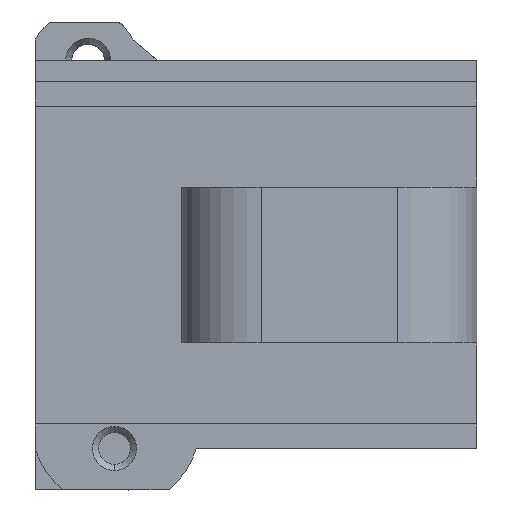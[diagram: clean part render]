
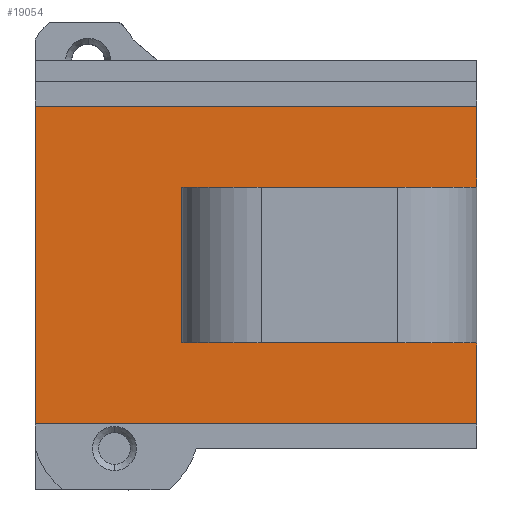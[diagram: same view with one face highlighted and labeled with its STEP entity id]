
A CAD part, left-side view. The second image highlights one B-rep face of the part: STEP entity #19054.
In plain terms, the highlighted planar face has unit normal (-1, 0, 0).
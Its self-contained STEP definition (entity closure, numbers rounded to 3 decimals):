
#2054 = DIRECTION ( 'NONE',  ( 0., 0., -1. ) ) ;
#2431 = VECTOR ( 'NONE', #35091, 1000. ) ;
#3809 = VERTEX_POINT ( 'NONE', #44843 ) ;
#7459 = LINE ( 'NONE', #10860, #109942 ) ;
#7646 = CARTESIAN_POINT ( 'NONE',  ( -40.849, 17.172, -13. ) ) ;
#8644 = DIRECTION ( 'NONE',  ( 0., 0., -1. ) ) ;
#9227 = EDGE_CURVE ( 'NONE', #20123, #62786, #75162, .T. ) ;
#9499 = VECTOR ( 'NONE', #72036, 1000. ) ;
#10860 = CARTESIAN_POINT ( 'NONE',  ( -40.849, 17.172, -13. ) ) ;
#11557 = ORIENTED_EDGE ( 'NONE', *, *, #70310, .F. ) ;
#17947 = VECTOR ( 'NONE', #8644, 1000. ) ;
#19054 = ADVANCED_FACE ( 'NONE', ( #81662 ), #106741, .F. ) ;
#19520 = CARTESIAN_POINT ( 'NONE',  ( -40.849, 53.322, -13. ) ) ;
#20123 = VERTEX_POINT ( 'NONE', #103717 ) ;
#20841 = EDGE_CURVE ( 'NONE', #71042, #84228, #68342, .T. ) ;
#23012 = CARTESIAN_POINT ( 'NONE',  ( -40.849, 17.172, -6.375 ) ) ;
#24553 = DIRECTION ( 'NONE',  ( 0., 1., 0. ) ) ;
#26527 = CARTESIAN_POINT ( 'NONE',  ( -40.849, 53.322, 6.375 ) ) ;
#31019 = CARTESIAN_POINT ( 'NONE',  ( -40.849, 17.172, -6.375 ) ) ;
#33047 = ORIENTED_EDGE ( 'NONE', *, *, #95310, .F. ) ;
#34868 = EDGE_CURVE ( 'NONE', #62786, #84228, #109665, .T. ) ;
#35056 = VECTOR ( 'NONE', #24553, 1000. ) ;
#35091 = DIRECTION ( 'NONE',  ( 0., 0., -1. ) ) ;
#36579 = DIRECTION ( 'NONE',  ( 0., 1., 0. ) ) ;
#37759 = CARTESIAN_POINT ( 'NONE',  ( -40.849, 17.172, 6.375 ) ) ;
#39074 = DIRECTION ( 'NONE',  ( 1., 0., 0. ) ) ;
#40991 = ORIENTED_EDGE ( 'NONE', *, *, #9227, .F. ) ;
#41283 = LINE ( 'NONE', #44464, #46621 ) ;
#41814 = LINE ( 'NONE', #100460, #35056 ) ;
#43015 = EDGE_CURVE ( 'NONE', #3809, #61138, #41814, .T. ) ;
#44464 = CARTESIAN_POINT ( 'NONE',  ( -40.849, 17.172, -9. ) ) ;
#44843 = CARTESIAN_POINT ( 'NONE',  ( -40.849, 17.172, 13. ) ) ;
#45579 = DIRECTION ( 'NONE',  ( 0., 1., 0. ) ) ;
#46569 = EDGE_LOOP ( 'NONE', ( #33047, #97140, #68248, #40991, #11557, #60206, #67529, #63967 ) ) ;
#46621 = VECTOR ( 'NONE', #2054, 1000. ) ;
#52796 = CARTESIAN_POINT ( 'NONE',  ( -40.849, 41.322, -6.375 ) ) ;
#56110 = CARTESIAN_POINT ( 'NONE',  ( -40.849, 41.322, -6.375 ) ) ;
#60094 = AXIS2_PLACEMENT_3D ( 'NONE', #65574, #39074, #90781 ) ;
#60206 = ORIENTED_EDGE ( 'NONE', *, *, #43015, .T. ) ;
#61138 = VERTEX_POINT ( 'NONE', #97646 ) ;
#62786 = VERTEX_POINT ( 'NONE', #106832 ) ;
#63967 = ORIENTED_EDGE ( 'NONE', *, *, #89012, .F. ) ;
#65574 = CARTESIAN_POINT ( 'NONE',  ( -40.849, 11.722, 6.375 ) ) ;
#67155 = VECTOR ( 'NONE', #45579, 1000. ) ;
#67440 = VERTEX_POINT ( 'NONE', #7646 ) ;
#67529 = ORIENTED_EDGE ( 'NONE', *, *, #104920, .T. ) ;
#68248 = ORIENTED_EDGE ( 'NONE', *, *, #34868, .F. ) ;
#68342 = LINE ( 'NONE', #31019, #9499 ) ;
#70310 = EDGE_CURVE ( 'NONE', #3809, #20123, #81019, .T. ) ;
#71042 = VERTEX_POINT ( 'NONE', #23012 ) ;
#72036 = DIRECTION ( 'NONE',  ( 0., 1., 0. ) ) ;
#75162 = LINE ( 'NONE', #37759, #67155 ) ;
#81019 = LINE ( 'NONE', #103536, #2431 ) ;
#81386 = DIRECTION ( 'NONE',  ( 0., 0., -1. ) ) ;
#81662 = FACE_OUTER_BOUND ( 'NONE', #46569, .T. ) ;
#84228 = VERTEX_POINT ( 'NONE', #52796 ) ;
#84429 = VECTOR ( 'NONE', #81386, 1000. ) ;
#88174 = VERTEX_POINT ( 'NONE', #19520 ) ;
#89012 = EDGE_CURVE ( 'NONE', #67440, #88174, #7459, .T. ) ;
#90781 = DIRECTION ( 'NONE',  ( 0., 0., -1. ) ) ;
#95310 = EDGE_CURVE ( 'NONE', #71042, #67440, #41283, .T. ) ;
#97140 = ORIENTED_EDGE ( 'NONE', *, *, #20841, .T. ) ;
#97646 = CARTESIAN_POINT ( 'NONE',  ( -40.849, 53.322, 13. ) ) ;
#100460 = CARTESIAN_POINT ( 'NONE',  ( -40.849, 17.172, 13. ) ) ;
#100538 = LINE ( 'NONE', #26527, #17947 ) ;
#103536 = CARTESIAN_POINT ( 'NONE',  ( -40.849, 17.172, -9. ) ) ;
#103717 = CARTESIAN_POINT ( 'NONE',  ( -40.849, 17.172, 6.375 ) ) ;
#104920 = EDGE_CURVE ( 'NONE', #61138, #88174, #100538, .T. ) ;
#106741 = PLANE ( 'NONE',  #60094 ) ;
#106832 = CARTESIAN_POINT ( 'NONE',  ( -40.849, 41.322, 6.375 ) ) ;
#109665 = LINE ( 'NONE', #56110, #84429 ) ;
#109942 = VECTOR ( 'NONE', #36579, 1000. ) ;
